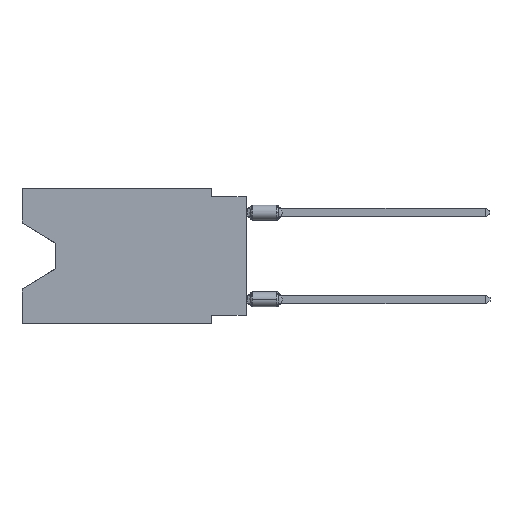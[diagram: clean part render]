
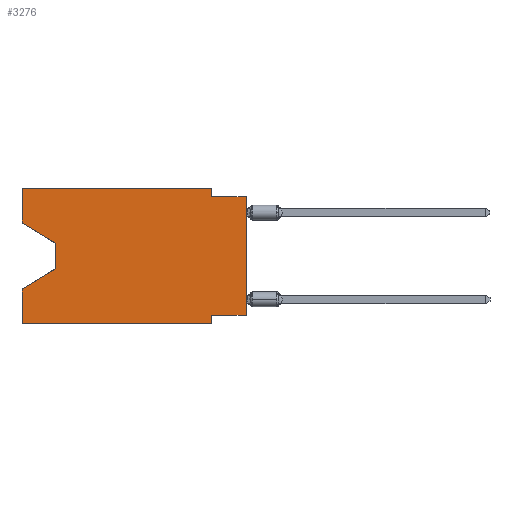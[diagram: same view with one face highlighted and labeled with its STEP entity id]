
A CAD part, left-side view. The second image highlights one B-rep face of the part: STEP entity #3276.
In plain terms, the highlighted planar face has unit normal (-1, 0, 0).
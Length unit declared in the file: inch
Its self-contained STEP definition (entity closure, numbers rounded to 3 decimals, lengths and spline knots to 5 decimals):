
#142 = CARTESIAN_POINT ( 'NONE',  ( 0., 0.1, -0.025 ) ) ;
#151 = VECTOR ( 'NONE', #3431, 39.37008 ) ;
#538 = VECTOR ( 'NONE', #7317, 39.37008 ) ;
#667 = EDGE_CURVE ( 'NONE', #7176, #18433, #15763, .T. ) ;
#935 = CARTESIAN_POINT ( 'NONE',  ( 0., 0., -0.365 ) ) ;
#1003 = CARTESIAN_POINT ( 'NONE',  ( 0., 0.1, 0. ) ) ;
#1154 = CARTESIAN_POINT ( 'NONE',  ( 0., 0.55, -0.232 ) ) ;
#1313 = CARTESIAN_POINT ( 'NONE',  ( 0., 0.645, -0.39 ) ) ;
#1565 = CARTESIAN_POINT ( 'NONE',  ( 0., 0.645, 0. ) ) ;
#1785 = LINE ( 'NONE', #1565, #3222 ) ;
#1837 = EDGE_CURVE ( 'NONE', #15382, #14549, #12180, .T. ) ;
#2205 = DIRECTION ( 'NONE',  ( 0., -0.855, -0.519 ) ) ;
#2227 = VECTOR ( 'NONE', #18890, 39.37008 ) ;
#2457 = VECTOR ( 'NONE', #9531, 39.37008 ) ;
#2999 = CARTESIAN_POINT ( 'NONE',  ( 0., 0.1, 0. ) ) ;
#3222 = VECTOR ( 'NONE', #16293, 39.37008 ) ;
#3276 = ADVANCED_FACE ( 'NONE', ( #16265 ), #8022, .F. ) ;
#3400 = CARTESIAN_POINT ( 'NONE',  ( 0., 0., -0.025 ) ) ;
#3431 = DIRECTION ( 'NONE',  ( 0., 0., 1. ) ) ;
#3464 = VERTEX_POINT ( 'NONE', #12554 ) ;
#3496 = VECTOR ( 'NONE', #15341, 39.37008 ) ;
#4265 = CARTESIAN_POINT ( 'NONE',  ( 0., 0.1, -0.39 ) ) ;
#4584 = EDGE_CURVE ( 'NONE', #5996, #11255, #1785, .T. ) ;
#4635 = EDGE_CURVE ( 'NONE', #8221, #3464, #13685, .T. ) ;
#4756 = VECTOR ( 'NONE', #19498, 39.37008 ) ;
#5155 = LINE ( 'NONE', #8507, #151 ) ;
#5261 = CARTESIAN_POINT ( 'NONE',  ( 0., 0.55, -0.232 ) ) ;
#5342 = EDGE_CURVE ( 'NONE', #8221, #5996, #5155, .T. ) ;
#5533 = ORIENTED_EDGE ( 'NONE', *, *, #5342, .F. ) ;
#5884 = CARTESIAN_POINT ( 'NONE',  ( 0., 0.1, -0.365 ) ) ;
#5948 = CARTESIAN_POINT ( 'NONE',  ( 0., 0.55, -0.158 ) ) ;
#5996 = VERTEX_POINT ( 'NONE', #14221 ) ;
#6006 = CARTESIAN_POINT ( 'NONE',  ( 0., 0.1, -0.39 ) ) ;
#7111 = LINE ( 'NONE', #935, #3496 ) ;
#7176 = VERTEX_POINT ( 'NONE', #5884 ) ;
#7190 = CARTESIAN_POINT ( 'NONE',  ( 0., 0.645, -0.10025 ) ) ;
#7224 = VECTOR ( 'NONE', #19644, 39.37008 ) ;
#7317 = DIRECTION ( 'NONE',  ( 0., 0.855, -0.519 ) ) ;
#7724 = EDGE_CURVE ( 'NONE', #11255, #14823, #17775, .T. ) ;
#8022 = PLANE ( 'NONE',  #8151 ) ;
#8151 = AXIS2_PLACEMENT_3D ( 'NONE', #14640, #14318, #11375 ) ;
#8193 = ORIENTED_EDGE ( 'NONE', *, *, #11520, .F. ) ;
#8221 = VERTEX_POINT ( 'NONE', #15706 ) ;
#8323 = DIRECTION ( 'NONE',  ( 0., -1., 0. ) ) ;
#8507 = CARTESIAN_POINT ( 'NONE',  ( 0., 0.645, 0. ) ) ;
#8523 = ORIENTED_EDGE ( 'NONE', *, *, #20557, .T. ) ;
#8856 = ORIENTED_EDGE ( 'NONE', *, *, #1837, .T. ) ;
#9049 = VERTEX_POINT ( 'NONE', #9854 ) ;
#9147 = ORIENTED_EDGE ( 'NONE', *, *, #7724, .F. ) ;
#9332 = VECTOR ( 'NONE', #19610, 39.37008 ) ;
#9398 = EDGE_CURVE ( 'NONE', #3464, #15382, #12882, .T. ) ;
#9531 = DIRECTION ( 'NONE',  ( 0., 0., -1. ) ) ;
#9617 = LINE ( 'NONE', #16240, #9332 ) ;
#9854 = CARTESIAN_POINT ( 'NONE',  ( 0., 0., -0.365 ) ) ;
#10500 = CARTESIAN_POINT ( 'NONE',  ( 0., 0.645, -0.39 ) ) ;
#10721 = VERTEX_POINT ( 'NONE', #10500 ) ;
#10736 = CARTESIAN_POINT ( 'NONE',  ( 0., 0., -0.025 ) ) ;
#11255 = VERTEX_POINT ( 'NONE', #2999 ) ;
#11375 = DIRECTION ( 'NONE',  ( 0., 0., -1. ) ) ;
#11395 = EDGE_LOOP ( 'NONE', ( #19016, #16158, #8856, #17207, #20017, #20762, #8193, #8523, #15443, #9147, #12490, #5533 ) ) ;
#11520 = EDGE_CURVE ( 'NONE', #9049, #7176, #7111, .T. ) ;
#12138 = EDGE_CURVE ( 'NONE', #10721, #18433, #19825, .T. ) ;
#12180 = LINE ( 'NONE', #5261, #538 ) ;
#12490 = ORIENTED_EDGE ( 'NONE', *, *, #4584, .F. ) ;
#12554 = CARTESIAN_POINT ( 'NONE',  ( 0., 0.55, -0.158 ) ) ;
#12882 = LINE ( 'NONE', #5948, #4756 ) ;
#13133 = LINE ( 'NONE', #16596, #7224 ) ;
#13685 = LINE ( 'NONE', #7190, #16712 ) ;
#14125 = VERTEX_POINT ( 'NONE', #3400 ) ;
#14221 = CARTESIAN_POINT ( 'NONE',  ( 0., 0.645, 0. ) ) ;
#14318 = DIRECTION ( 'NONE',  ( 1., 0., 0. ) ) ;
#14549 = VERTEX_POINT ( 'NONE', #20711 ) ;
#14640 = CARTESIAN_POINT ( 'NONE',  ( 0., 0.645, 0. ) ) ;
#14823 = VERTEX_POINT ( 'NONE', #142 ) ;
#15341 = DIRECTION ( 'NONE',  ( 0., 1., 0. ) ) ;
#15382 = VERTEX_POINT ( 'NONE', #1154 ) ;
#15443 = ORIENTED_EDGE ( 'NONE', *, *, #21312, .F. ) ;
#15706 = CARTESIAN_POINT ( 'NONE',  ( 0., 0.645, -0.10025 ) ) ;
#15763 = LINE ( 'NONE', #6006, #2227 ) ;
#16158 = ORIENTED_EDGE ( 'NONE', *, *, #9398, .T. ) ;
#16240 = CARTESIAN_POINT ( 'NONE',  ( 0., 0., 0. ) ) ;
#16265 = FACE_OUTER_BOUND ( 'NONE', #11395, .T. ) ;
#16293 = DIRECTION ( 'NONE',  ( 0., -1., 0. ) ) ;
#16596 = CARTESIAN_POINT ( 'NONE',  ( 0., 0.645, 0. ) ) ;
#16712 = VECTOR ( 'NONE', #2205, 39.37008 ) ;
#17179 = EDGE_CURVE ( 'NONE', #10721, #14549, #13133, .T. ) ;
#17207 = ORIENTED_EDGE ( 'NONE', *, *, #17179, .F. ) ;
#17363 = DIRECTION ( 'NONE',  ( 0., -1., 0. ) ) ;
#17673 = VECTOR ( 'NONE', #17363, 39.37008 ) ;
#17775 = LINE ( 'NONE', #1003, #2457 ) ;
#18433 = VERTEX_POINT ( 'NONE', #4265 ) ;
#18890 = DIRECTION ( 'NONE',  ( 0., 0., -1. ) ) ;
#19016 = ORIENTED_EDGE ( 'NONE', *, *, #4635, .T. ) ;
#19198 = LINE ( 'NONE', #10736, #17673 ) ;
#19498 = DIRECTION ( 'NONE',  ( 0., 0., -1. ) ) ;
#19610 = DIRECTION ( 'NONE',  ( 0., 0., 1. ) ) ;
#19644 = DIRECTION ( 'NONE',  ( 0., 0., 1. ) ) ;
#19825 = LINE ( 'NONE', #1313, #20119 ) ;
#20017 = ORIENTED_EDGE ( 'NONE', *, *, #12138, .T. ) ;
#20119 = VECTOR ( 'NONE', #8323, 39.37008 ) ;
#20557 = EDGE_CURVE ( 'NONE', #9049, #14125, #9617, .T. ) ;
#20711 = CARTESIAN_POINT ( 'NONE',  ( 0., 0.645, -0.28975 ) ) ;
#20762 = ORIENTED_EDGE ( 'NONE', *, *, #667, .F. ) ;
#21312 = EDGE_CURVE ( 'NONE', #14823, #14125, #19198, .T. ) ;
